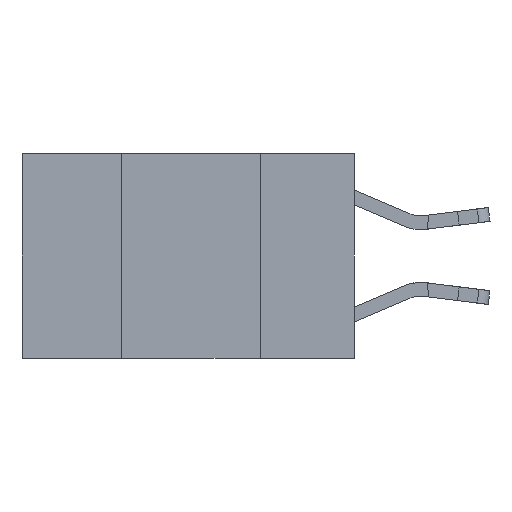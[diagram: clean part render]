
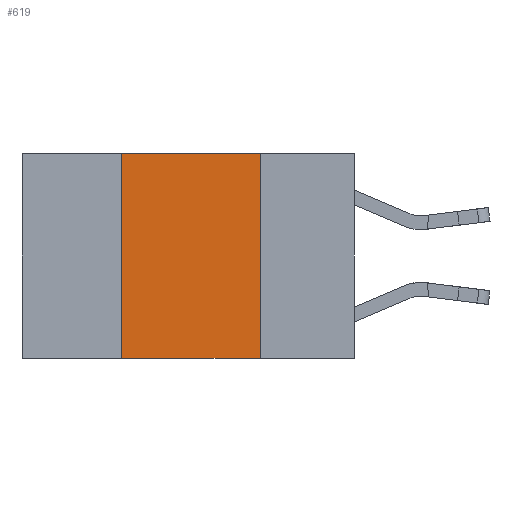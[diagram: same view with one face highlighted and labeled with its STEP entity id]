
A CAD part, left-side view. The second image highlights one B-rep face of the part: STEP entity #619.
In plain terms, the highlighted planar face has unit normal (-1, 0, 0).
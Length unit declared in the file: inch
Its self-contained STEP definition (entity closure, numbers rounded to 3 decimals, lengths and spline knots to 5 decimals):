
#619 = ADVANCED_FACE ( 'NONE', ( #15907 ), #4752, .F. ) ;
#1234 = VERTEX_POINT ( 'NONE', #3452 ) ;
#3452 = CARTESIAN_POINT ( 'NONE',  ( 0., 0.42, -0.37 ) ) ;
#4088 = ORIENTED_EDGE ( 'NONE', *, *, #8590, .F. ) ;
#4752 = PLANE ( 'NONE',  #8492 ) ;
#5503 = EDGE_CURVE ( 'NONE', #1234, #8495, #9614, .T. ) ;
#5914 = CARTESIAN_POINT ( 'NONE',  ( 0., 0.17, -0.37 ) ) ;
#6041 = VECTOR ( 'NONE', #16890, 39.37008 ) ;
#6441 = EDGE_CURVE ( 'NONE', #1234, #16124, #7139, .T. ) ;
#6573 = VECTOR ( 'NONE', #12764, 39.37008 ) ;
#6647 = CARTESIAN_POINT ( 'NONE',  ( 0., 0.17, 0. ) ) ;
#6831 = CARTESIAN_POINT ( 'NONE',  ( 0., 0.6, 0. ) ) ;
#7139 = LINE ( 'NONE', #17107, #6573 ) ;
#7687 = ORIENTED_EDGE ( 'NONE', *, *, #14426, .F. ) ;
#8492 = AXIS2_PLACEMENT_3D ( 'NONE', #11660, #15812, #10371 ) ;
#8495 = VERTEX_POINT ( 'NONE', #15324 ) ;
#8590 = EDGE_CURVE ( 'NONE', #8495, #13205, #12724, .T. ) ;
#9614 = LINE ( 'NONE', #16721, #11808 ) ;
#9667 = ORIENTED_EDGE ( 'NONE', *, *, #5503, .F. ) ;
#10365 = DIRECTION ( 'NONE',  ( 0., 0., -1. ) ) ;
#10371 = DIRECTION ( 'NONE',  ( 0., 0., -1. ) ) ;
#11660 = CARTESIAN_POINT ( 'NONE',  ( 0., 0.6, 0. ) ) ;
#11808 = VECTOR ( 'NONE', #13768, 39.37008 ) ;
#12724 = LINE ( 'NONE', #6831, #6041 ) ;
#12764 = DIRECTION ( 'NONE',  ( 0., -1., 0. ) ) ;
#13205 = VERTEX_POINT ( 'NONE', #6647 ) ;
#13223 = VECTOR ( 'NONE', #10365, 39.37008 ) ;
#13768 = DIRECTION ( 'NONE',  ( 0., 0., 1. ) ) ;
#14426 = EDGE_CURVE ( 'NONE', #13205, #16124, #14884, .T. ) ;
#14884 = LINE ( 'NONE', #17640, #13223 ) ;
#15324 = CARTESIAN_POINT ( 'NONE',  ( 0., 0.42, 0. ) ) ;
#15812 = DIRECTION ( 'NONE',  ( 1., 0., 0. ) ) ;
#15907 = FACE_OUTER_BOUND ( 'NONE', #16690, .T. ) ;
#16124 = VERTEX_POINT ( 'NONE', #5914 ) ;
#16148 = ORIENTED_EDGE ( 'NONE', *, *, #6441, .T. ) ;
#16690 = EDGE_LOOP ( 'NONE', ( #7687, #4088, #9667, #16148 ) ) ;
#16721 = CARTESIAN_POINT ( 'NONE',  ( 0., 0.42, 0. ) ) ;
#16890 = DIRECTION ( 'NONE',  ( 0., -1., 0. ) ) ;
#17107 = CARTESIAN_POINT ( 'NONE',  ( 0., 0.6, -0.37 ) ) ;
#17640 = CARTESIAN_POINT ( 'NONE',  ( 0., 0.17, 0. ) ) ;
